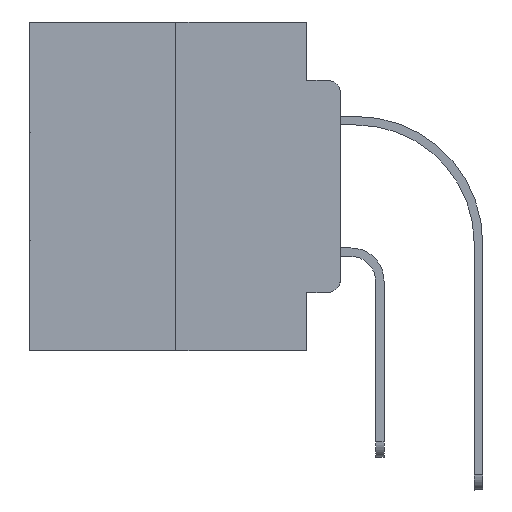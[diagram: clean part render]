
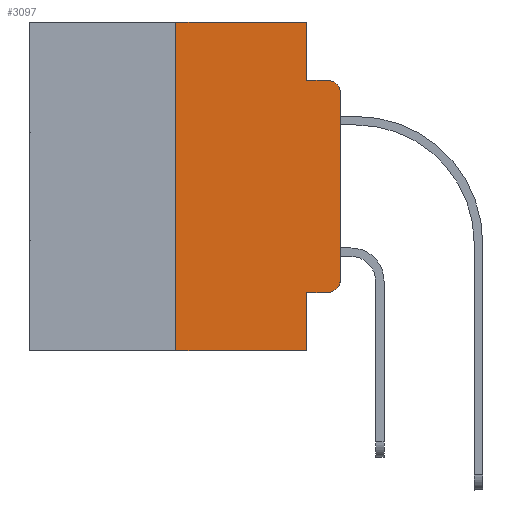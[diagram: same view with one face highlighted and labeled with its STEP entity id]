
A CAD part, left-side view. The second image highlights one B-rep face of the part: STEP entity #3097.
In plain terms, the highlighted planar face has unit normal (-1, 0, 0).
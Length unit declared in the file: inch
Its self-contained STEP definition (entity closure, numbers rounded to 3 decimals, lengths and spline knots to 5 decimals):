
#75 = FACE_OUTER_BOUND ( 'NONE', #10503, .T. ) ;
#2242 = VECTOR ( 'NONE', #20732, 39.37008 ) ;
#2281 = LINE ( 'NONE', #13960, #2242 ) ;
#2594 = ORIENTED_EDGE ( 'NONE', *, *, #25830, .T. ) ;
#2688 = AXIS2_PLACEMENT_3D ( 'NONE', #28207, #7007, #4389 ) ;
#3097 = ADVANCED_FACE ( 'NONE', ( #75 ), #9586, .F. ) ;
#3223 = EDGE_CURVE ( 'NONE', #29962, #23128, #19857, .T. ) ;
#3455 = EDGE_CURVE ( 'NONE', #4576, #26268, #18179, .T. ) ;
#3488 = LINE ( 'NONE', #24698, #29138 ) ;
#4198 = DIRECTION ( 'NONE',  ( 0., -1., 0. ) ) ;
#4389 = DIRECTION ( 'NONE',  ( 0., 0., -1. ) ) ;
#4576 = VERTEX_POINT ( 'NONE', #10504 ) ;
#4592 = DIRECTION ( 'NONE',  ( 0., 0., -1. ) ) ;
#5314 = CARTESIAN_POINT ( 'NONE',  ( 0., 0.051, 0. ) ) ;
#7007 = DIRECTION ( 'NONE',  ( 1., 0., 0. ) ) ;
#8164 = VECTOR ( 'NONE', #23374, 39.37008 ) ;
#8237 = VERTEX_POINT ( 'NONE', #22843 ) ;
#8462 = CARTESIAN_POINT ( 'NONE',  ( 0., 0., -0.1085 ) ) ;
#8710 = DIRECTION ( 'NONE',  ( 0., -1., 0. ) ) ;
#8849 = ORIENTED_EDGE ( 'NONE', *, *, #19112, .T. ) ;
#9240 = CARTESIAN_POINT ( 'NONE',  ( 0., 0.25, 0. ) ) ;
#9586 = PLANE ( 'NONE',  #2688 ) ;
#10503 = EDGE_LOOP ( 'NONE', ( #24894, #15453, #29930, #14740, #21945, #22830, #2594, #21080, #8849, #16744 ) ) ;
#10504 = CARTESIAN_POINT ( 'NONE',  ( 0., 0.051, -0.0885 ) ) ;
#11500 = VECTOR ( 'NONE', #13176, 39.37008 ) ;
#12641 = VECTOR ( 'NONE', #25355, 39.37008 ) ;
#13024 = LINE ( 'NONE', #22388, #11500 ) ;
#13176 = DIRECTION ( 'NONE',  ( 0., 0., -1. ) ) ;
#13222 = EDGE_CURVE ( 'NONE', #23128, #19414, #19520, .T. ) ;
#13482 = VECTOR ( 'NONE', #4198, 39.37008 ) ;
#13789 = EDGE_CURVE ( 'NONE', #8237, #17861, #13024, .T. ) ;
#13960 = CARTESIAN_POINT ( 'NONE',  ( 0., 0.473, -0.5 ) ) ;
#13996 = LINE ( 'NONE', #19069, #8164 ) ;
#14494 = DIRECTION ( 'NONE',  ( -1., 0., 0. ) ) ;
#14691 = EDGE_CURVE ( 'NONE', #29349, #15997, #3488, .T. ) ;
#14740 = ORIENTED_EDGE ( 'NONE', *, *, #26723, .F. ) ;
#15453 = ORIENTED_EDGE ( 'NONE', *, *, #25828, .T. ) ;
#15875 = VECTOR ( 'NONE', #8710, 39.37008 ) ;
#15997 = VERTEX_POINT ( 'NONE', #9240 ) ;
#16103 = DIRECTION ( 'NONE',  ( -1., 0., 0. ) ) ;
#16401 = CARTESIAN_POINT ( 'NONE',  ( 0., 0.02, -0.1085 ) ) ;
#16744 = ORIENTED_EDGE ( 'NONE', *, *, #3223, .T. ) ;
#17145 = VECTOR ( 'NONE', #27411, 39.37008 ) ;
#17861 = VERTEX_POINT ( 'NONE', #28427 ) ;
#18179 = LINE ( 'NONE', #27575, #13482 ) ;
#19069 = CARTESIAN_POINT ( 'NONE',  ( 0., 0.051, 0. ) ) ;
#19100 = CARTESIAN_POINT ( 'NONE',  ( 0., 0.02, -0.0885 ) ) ;
#19112 = EDGE_CURVE ( 'NONE', #8237, #29962, #27868, .T. ) ;
#19354 = AXIS2_PLACEMENT_3D ( 'NONE', #24033, #14494, #22035 ) ;
#19414 = VERTEX_POINT ( 'NONE', #8462 ) ;
#19520 = LINE ( 'NONE', #28913, #12641 ) ;
#19857 = CIRCLE ( 'NONE', #19354, 0.02 ) ;
#20539 = LINE ( 'NONE', #29777, #15875 ) ;
#20635 = CARTESIAN_POINT ( 'NONE',  ( 0., 0.051, -0.4115 ) ) ;
#20732 = DIRECTION ( 'NONE',  ( 0., -1., 0. ) ) ;
#21080 = ORIENTED_EDGE ( 'NONE', *, *, #13789, .F. ) ;
#21939 = CIRCLE ( 'NONE', #27278, 0.02 ) ;
#21945 = ORIENTED_EDGE ( 'NONE', *, *, #22723, .F. ) ;
#22035 = DIRECTION ( 'NONE',  ( 0., 0., -1. ) ) ;
#22388 = CARTESIAN_POINT ( 'NONE',  ( 0., 0.051, 0. ) ) ;
#22704 = CARTESIAN_POINT ( 'NONE',  ( 0., 0.02, -0.4115 ) ) ;
#22723 = EDGE_CURVE ( 'NONE', #15997, #28584, #20539, .T. ) ;
#22830 = ORIENTED_EDGE ( 'NONE', *, *, #14691, .F. ) ;
#22843 = CARTESIAN_POINT ( 'NONE',  ( 0., 0.051, -0.4115 ) ) ;
#23128 = VERTEX_POINT ( 'NONE', #25461 ) ;
#23374 = DIRECTION ( 'NONE',  ( 0., 0., -1. ) ) ;
#24033 = CARTESIAN_POINT ( 'NONE',  ( 0., 0.02, -0.3915 ) ) ;
#24698 = CARTESIAN_POINT ( 'NONE',  ( 0., 0.25, 0. ) ) ;
#24894 = ORIENTED_EDGE ( 'NONE', *, *, #13222, .T. ) ;
#25355 = DIRECTION ( 'NONE',  ( 0., 0., 1. ) ) ;
#25461 = CARTESIAN_POINT ( 'NONE',  ( 0., 0., -0.3915 ) ) ;
#25828 = EDGE_CURVE ( 'NONE', #19414, #26268, #21939, .T. ) ;
#25830 = EDGE_CURVE ( 'NONE', #29349, #17861, #2281, .T. ) ;
#26268 = VERTEX_POINT ( 'NONE', #19100 ) ;
#26723 = EDGE_CURVE ( 'NONE', #28584, #4576, #13996, .T. ) ;
#27157 = DIRECTION ( 'NONE',  ( 0., 0., 1. ) ) ;
#27278 = AXIS2_PLACEMENT_3D ( 'NONE', #16401, #16103, #4592 ) ;
#27411 = DIRECTION ( 'NONE',  ( 0., -1., 0. ) ) ;
#27575 = CARTESIAN_POINT ( 'NONE',  ( 0., 0.051, -0.0885 ) ) ;
#27868 = LINE ( 'NONE', #20635, #17145 ) ;
#28207 = CARTESIAN_POINT ( 'NONE',  ( 0., 0.473, 0. ) ) ;
#28427 = CARTESIAN_POINT ( 'NONE',  ( 0., 0.051, -0.5 ) ) ;
#28584 = VERTEX_POINT ( 'NONE', #5314 ) ;
#28913 = CARTESIAN_POINT ( 'NONE',  ( 0., 0., 0. ) ) ;
#29138 = VECTOR ( 'NONE', #27157, 39.37008 ) ;
#29349 = VERTEX_POINT ( 'NONE', #30325 ) ;
#29777 = CARTESIAN_POINT ( 'NONE',  ( 0., 0.473, 0. ) ) ;
#29930 = ORIENTED_EDGE ( 'NONE', *, *, #3455, .F. ) ;
#29962 = VERTEX_POINT ( 'NONE', #22704 ) ;
#30325 = CARTESIAN_POINT ( 'NONE',  ( 0., 0.25, -0.5 ) ) ;
